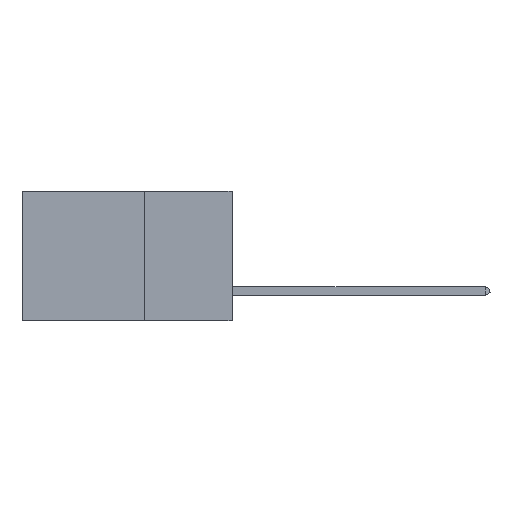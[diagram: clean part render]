
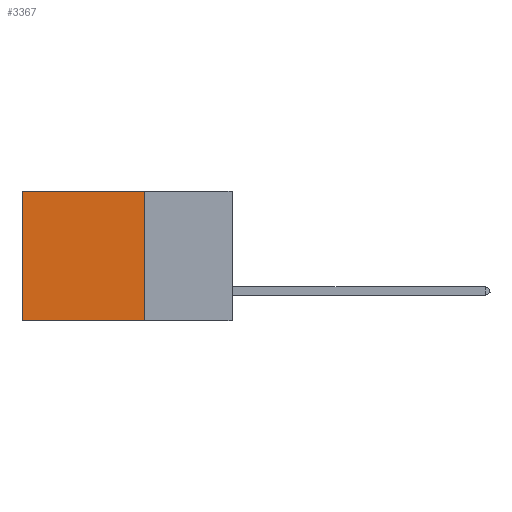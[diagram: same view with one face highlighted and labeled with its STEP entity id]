
A CAD part, left-side view. The second image highlights one B-rep face of the part: STEP entity #3367.
In plain terms, the highlighted planar face has unit normal (-1, 0, 0).
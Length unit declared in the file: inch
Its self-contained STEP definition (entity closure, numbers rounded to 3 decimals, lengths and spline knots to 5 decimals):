
#937 = EDGE_LOOP ( 'NONE', ( #15940, #12755, #5146, #11573 ) ) ;
#1294 = CARTESIAN_POINT ( 'NONE',  ( 0.2875, 0.25, -0.37 ) ) ;
#1854 = CARTESIAN_POINT ( 'NONE',  ( 0.2875, 0.6, 0. ) ) ;
#2412 = EDGE_CURVE ( 'NONE', #10649, #11827, #13365, .T. ) ;
#3294 = LINE ( 'NONE', #6199, #8905 ) ;
#3367 = ADVANCED_FACE ( 'NONE', ( #15050 ), #10812, .F. ) ;
#3719 = DIRECTION ( 'NONE',  ( 0., 0., -1. ) ) ;
#4620 = LINE ( 'NONE', #10229, #13835 ) ;
#4638 = DIRECTION ( 'NONE',  ( 1., 0., 0. ) ) ;
#4809 = DIRECTION ( 'NONE',  ( 0., 0., -1. ) ) ;
#5146 = ORIENTED_EDGE ( 'NONE', *, *, #15728, .F. ) ;
#5664 = DIRECTION ( 'NONE',  ( 0., 1., 0. ) ) ;
#6199 = CARTESIAN_POINT ( 'NONE',  ( 0.2875, 0.6, 0. ) ) ;
#6717 = VECTOR ( 'NONE', #15656, 39.37008 ) ;
#7583 = EDGE_CURVE ( 'NONE', #14843, #9214, #4620, .T. ) ;
#8074 = CARTESIAN_POINT ( 'NONE',  ( 0.2875, 0.25, -0.37 ) ) ;
#8466 = CARTESIAN_POINT ( 'NONE',  ( 0.2875, 0.25, 0. ) ) ;
#8905 = VECTOR ( 'NONE', #3719, 39.37008 ) ;
#9214 = VERTEX_POINT ( 'NONE', #1854 ) ;
#9837 = AXIS2_PLACEMENT_3D ( 'NONE', #8466, #4638, #4809 ) ;
#10229 = CARTESIAN_POINT ( 'NONE',  ( 0.2875, 0.25, 0. ) ) ;
#10438 = CARTESIAN_POINT ( 'NONE',  ( 0.2875, 0.25, 0. ) ) ;
#10649 = VERTEX_POINT ( 'NONE', #1294 ) ;
#10812 = PLANE ( 'NONE',  #9837 ) ;
#10907 = CARTESIAN_POINT ( 'NONE',  ( 0.2875, 0.25, 0. ) ) ;
#11573 = ORIENTED_EDGE ( 'NONE', *, *, #7583, .T. ) ;
#11827 = VERTEX_POINT ( 'NONE', #12210 ) ;
#12210 = CARTESIAN_POINT ( 'NONE',  ( 0.2875, 0.6, -0.37 ) ) ;
#12755 = ORIENTED_EDGE ( 'NONE', *, *, #2412, .F. ) ;
#13174 = VECTOR ( 'NONE', #15433, 39.37008 ) ;
#13217 = LINE ( 'NONE', #10438, #6717 ) ;
#13365 = LINE ( 'NONE', #8074, #13174 ) ;
#13835 = VECTOR ( 'NONE', #5664, 39.37008 ) ;
#14133 = EDGE_CURVE ( 'NONE', #9214, #11827, #3294, .T. ) ;
#14843 = VERTEX_POINT ( 'NONE', #10907 ) ;
#15050 = FACE_OUTER_BOUND ( 'NONE', #937, .T. ) ;
#15433 = DIRECTION ( 'NONE',  ( 0., 1., 0. ) ) ;
#15656 = DIRECTION ( 'NONE',  ( 0., 0., -1. ) ) ;
#15728 = EDGE_CURVE ( 'NONE', #14843, #10649, #13217, .T. ) ;
#15940 = ORIENTED_EDGE ( 'NONE', *, *, #14133, .T. ) ;
